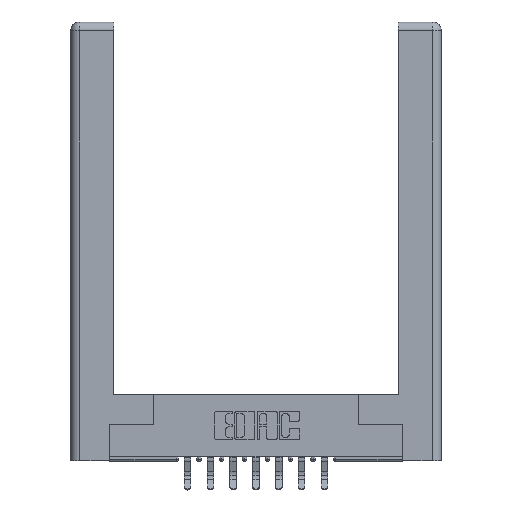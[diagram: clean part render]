
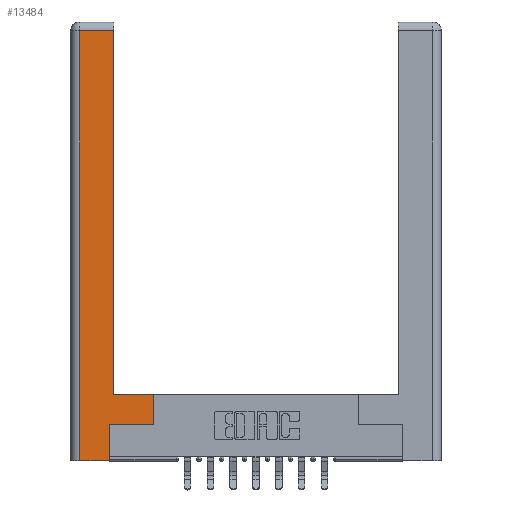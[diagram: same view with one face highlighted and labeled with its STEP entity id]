
A CAD part, top view. The second image highlights one B-rep face of the part: STEP entity #13484.
In plain terms, the highlighted planar face has unit normal (0, 0, 1).
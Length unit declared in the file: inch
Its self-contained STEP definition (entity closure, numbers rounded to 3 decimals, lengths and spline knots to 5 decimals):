
#346 = LINE ( 'NONE', #5232, #2285 ) ;
#528 = CARTESIAN_POINT ( 'NONE',  ( 0.265, 0.245, 0. ) ) ;
#1448 = EDGE_CURVE ( 'NONE', #11319, #4835, #346, .T. ) ;
#1783 = AXIS2_PLACEMENT_3D ( 'NONE', #1900, #3732, #11653 ) ;
#1900 = CARTESIAN_POINT ( 'NONE',  ( 0., 0., 0. ) ) ;
#2070 = CARTESIAN_POINT ( 'NONE',  ( 0.265, 0.245, 0. ) ) ;
#2259 = VECTOR ( 'NONE', #2365, 39.37008 ) ;
#2285 = VECTOR ( 'NONE', #4124, 39.37008 ) ;
#2365 = DIRECTION ( 'NONE',  ( 0., 1., 0. ) ) ;
#2402 = CARTESIAN_POINT ( 'NONE',  ( 0.265, 0., 0. ) ) ;
#2512 = CARTESIAN_POINT ( 'NONE',  ( 0.0615, 0., 0. ) ) ;
#2780 = EDGE_LOOP ( 'NONE', ( #11236, #7127, #2993, #6819, #13902, #3423, #5295, #12558 ) ) ;
#2993 = ORIENTED_EDGE ( 'NONE', *, *, #14121, .T. ) ;
#3127 = LINE ( 'NONE', #2512, #3469 ) ;
#3160 = CARTESIAN_POINT ( 'NONE',  ( 0.265, 0., 0. ) ) ;
#3423 = ORIENTED_EDGE ( 'NONE', *, *, #1448, .T. ) ;
#3451 = VERTEX_POINT ( 'NONE', #8796 ) ;
#3469 = VECTOR ( 'NONE', #4581, 39.37008 ) ;
#3498 = VERTEX_POINT ( 'NONE', #2402 ) ;
#3732 = DIRECTION ( 'NONE',  ( 0., 0., -1. ) ) ;
#3749 = VERTEX_POINT ( 'NONE', #5893 ) ;
#4124 = DIRECTION ( 'NONE',  ( 1., 0., 0. ) ) ;
#4581 = DIRECTION ( 'NONE',  ( 0., -1., 0. ) ) ;
#4761 = DIRECTION ( 'NONE',  ( 0., 1., 0. ) ) ;
#4835 = VERTEX_POINT ( 'NONE', #6567 ) ;
#5006 = DIRECTION ( 'NONE',  ( 0., 1., 0. ) ) ;
#5232 = CARTESIAN_POINT ( 'NONE',  ( 0.565, 0.245, 0. ) ) ;
#5295 = ORIENTED_EDGE ( 'NONE', *, *, #11122, .T. ) ;
#5527 = CARTESIAN_POINT ( 'NONE',  ( 0.565, 0.45, 0. ) ) ;
#5646 = LINE ( 'NONE', #8372, #14582 ) ;
#5763 = CARTESIAN_POINT ( 'NONE',  ( 0.295, 3., 0. ) ) ;
#5893 = CARTESIAN_POINT ( 'NONE',  ( 0.295, 0.45, 0. ) ) ;
#6074 = PLANE ( 'NONE',  #1783 ) ;
#6097 = DIRECTION ( 'NONE',  ( -1., 0., 0. ) ) ;
#6444 = VECTOR ( 'NONE', #4761, 39.37008 ) ;
#6532 = DIRECTION ( 'NONE',  ( 1., 0., 0. ) ) ;
#6567 = CARTESIAN_POINT ( 'NONE',  ( 0.565, 0.245, 0. ) ) ;
#6623 = LINE ( 'NONE', #14043, #6444 ) ;
#6818 = DIRECTION ( 'NONE',  ( -1., 0., 0. ) ) ;
#6819 = ORIENTED_EDGE ( 'NONE', *, *, #13509, .T. ) ;
#6836 = FACE_OUTER_BOUND ( 'NONE', #2780, .T. ) ;
#7127 = ORIENTED_EDGE ( 'NONE', *, *, #7628, .T. ) ;
#7628 = EDGE_CURVE ( 'NONE', #13689, #14010, #5646, .T. ) ;
#7665 = EDGE_CURVE ( 'NONE', #3498, #11319, #7946, .T. ) ;
#7946 = LINE ( 'NONE', #528, #8493 ) ;
#8372 = CARTESIAN_POINT ( 'NONE',  ( 0.0615, 2.94, 0. ) ) ;
#8493 = VECTOR ( 'NONE', #5006, 39.37008 ) ;
#8796 = CARTESIAN_POINT ( 'NONE',  ( 0.0615, 0., 0. ) ) ;
#8983 = VECTOR ( 'NONE', #6818, 39.37008 ) ;
#9151 = LINE ( 'NONE', #3160, #10618 ) ;
#9340 = LINE ( 'NONE', #11315, #8983 ) ;
#10618 = VECTOR ( 'NONE', #6532, 39.37008 ) ;
#11122 = EDGE_CURVE ( 'NONE', #4835, #11648, #6623, .T. ) ;
#11236 = ORIENTED_EDGE ( 'NONE', *, *, #13367, .T. ) ;
#11315 = CARTESIAN_POINT ( 'NONE',  ( 0.295, 0.45, 0. ) ) ;
#11319 = VERTEX_POINT ( 'NONE', #2070 ) ;
#11648 = VERTEX_POINT ( 'NONE', #5527 ) ;
#11653 = DIRECTION ( 'NONE',  ( -1., 0., 0. ) ) ;
#12375 = CARTESIAN_POINT ( 'NONE',  ( 0.0615, 2.94, 0. ) ) ;
#12558 = ORIENTED_EDGE ( 'NONE', *, *, #13182, .T. ) ;
#12923 = LINE ( 'NONE', #5763, #2259 ) ;
#13182 = EDGE_CURVE ( 'NONE', #11648, #3749, #9340, .T. ) ;
#13367 = EDGE_CURVE ( 'NONE', #3749, #13689, #12923, .T. ) ;
#13484 = ADVANCED_FACE ( 'NONE', ( #6836 ), #6074, .F. ) ;
#13509 = EDGE_CURVE ( 'NONE', #3451, #3498, #9151, .T. ) ;
#13638 = CARTESIAN_POINT ( 'NONE',  ( 0.295, 2.94, 0. ) ) ;
#13689 = VERTEX_POINT ( 'NONE', #13638 ) ;
#13902 = ORIENTED_EDGE ( 'NONE', *, *, #7665, .T. ) ;
#14010 = VERTEX_POINT ( 'NONE', #12375 ) ;
#14043 = CARTESIAN_POINT ( 'NONE',  ( 0.565, 0.45, 0. ) ) ;
#14121 = EDGE_CURVE ( 'NONE', #14010, #3451, #3127, .T. ) ;
#14582 = VECTOR ( 'NONE', #6097, 39.37008 ) ;
